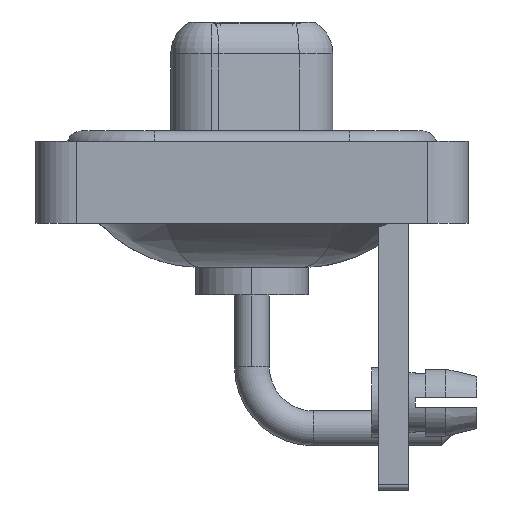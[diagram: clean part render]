
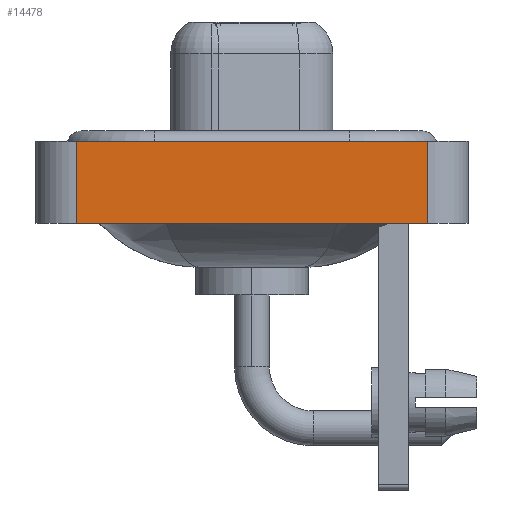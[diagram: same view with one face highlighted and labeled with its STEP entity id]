
A CAD part, left-side view. The second image highlights one B-rep face of the part: STEP entity #14478.
In plain terms, the highlighted planar face has unit normal (-1, 0, 0).
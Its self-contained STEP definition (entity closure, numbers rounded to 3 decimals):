
#207 = ORIENTED_EDGE ( 'NONE', *, *, #17358, .F. ) ;
#820 = LINE ( 'NONE', #16464, #15858 ) ;
#1578 = EDGE_LOOP ( 'NONE', ( #8043, #5743, #207, #8014 ) ) ;
#2251 = CARTESIAN_POINT ( 'NONE',  ( -7.3, -8.55, -3.6 ) ) ;
#2345 = DIRECTION ( 'NONE',  ( -1., 0., 0. ) ) ;
#2389 = CARTESIAN_POINT ( 'NONE',  ( -7.3, -8.55, -3.6 ) ) ;
#2441 = CARTESIAN_POINT ( 'NONE',  ( -7.3, -8.55, 0.4 ) ) ;
#2794 = DIRECTION ( 'NONE',  ( 0., -1., 0. ) ) ;
#3681 = LINE ( 'NONE', #15113, #3855 ) ;
#3855 = VECTOR ( 'NONE', #13619, 1000. ) ;
#4807 = EDGE_CURVE ( 'NONE', #7145, #15714, #18343, .T. ) ;
#5213 = EDGE_CURVE ( 'NONE', #18196, #15714, #15221, .T. ) ;
#5743 = ORIENTED_EDGE ( 'NONE', *, *, #4807, .F. ) ;
#6946 = CARTESIAN_POINT ( 'NONE',  ( -7.3, -8.55, 0.4 ) ) ;
#6991 = EDGE_CURVE ( 'NONE', #18466, #18196, #3681, .T. ) ;
#7145 = VERTEX_POINT ( 'NONE', #12769 ) ;
#7566 = VECTOR ( 'NONE', #2794, 1000. ) ;
#8014 = ORIENTED_EDGE ( 'NONE', *, *, #6991, .T. ) ;
#8043 = ORIENTED_EDGE ( 'NONE', *, *, #5213, .T. ) ;
#8113 = DIRECTION ( 'NONE',  ( 0., 0., 1. ) ) ;
#9286 = DIRECTION ( 'NONE',  ( 0., 0., 1. ) ) ;
#10078 = AXIS2_PLACEMENT_3D ( 'NONE', #2251, #2345, #13686 ) ;
#10778 = FACE_OUTER_BOUND ( 'NONE', #1578, .T. ) ;
#10812 = CARTESIAN_POINT ( 'NONE',  ( -7.3, 8.55, -3.6 ) ) ;
#11301 = CARTESIAN_POINT ( 'NONE',  ( -7.3, -8.55, -3.6 ) ) ;
#12769 = CARTESIAN_POINT ( 'NONE',  ( -7.3, 8.55, 0.4 ) ) ;
#13619 = DIRECTION ( 'NONE',  ( 0., -1., 0. ) ) ;
#13686 = DIRECTION ( 'NONE',  ( 0., 0., 1. ) ) ;
#14448 = VECTOR ( 'NONE', #8113, 1000. ) ;
#14478 = ADVANCED_FACE ( 'NONE', ( #10778 ), #16478, .T. ) ;
#15113 = CARTESIAN_POINT ( 'NONE',  ( -7.3, -8.55, -3.6 ) ) ;
#15221 = LINE ( 'NONE', #2389, #14448 ) ;
#15714 = VERTEX_POINT ( 'NONE', #2441 ) ;
#15858 = VECTOR ( 'NONE', #9286, 1000. ) ;
#16464 = CARTESIAN_POINT ( 'NONE',  ( -7.3, 8.55, -3.6 ) ) ;
#16478 = PLANE ( 'NONE',  #10078 ) ;
#17358 = EDGE_CURVE ( 'NONE', #18466, #7145, #820, .T. ) ;
#18196 = VERTEX_POINT ( 'NONE', #11301 ) ;
#18343 = LINE ( 'NONE', #6946, #7566 ) ;
#18466 = VERTEX_POINT ( 'NONE', #10812 ) ;
